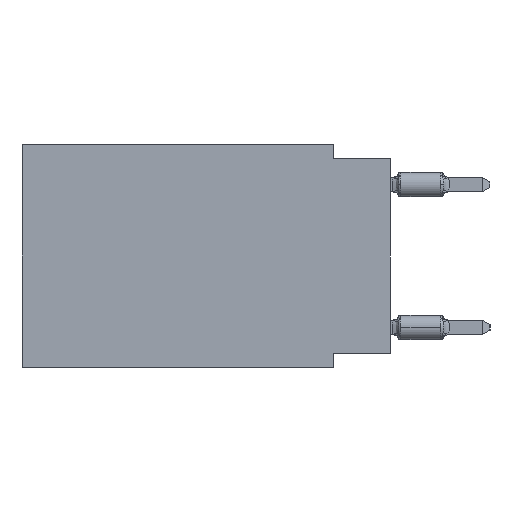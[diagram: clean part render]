
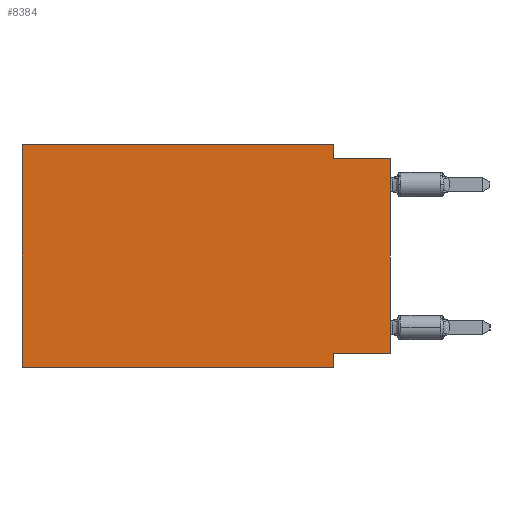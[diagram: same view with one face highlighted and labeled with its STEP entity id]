
A CAD part, left-side view. The second image highlights one B-rep face of the part: STEP entity #8384.
In plain terms, the highlighted planar face has unit normal (-1, 0, 0).
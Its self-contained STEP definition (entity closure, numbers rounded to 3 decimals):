
#720 = CARTESIAN_POINT ( 'NONE',  ( 0., 16.383, 0. ) ) ;
#1189 = VERTEX_POINT ( 'NONE', #13962 ) ;
#1485 = ORIENTED_EDGE ( 'NONE', *, *, #22149, .F. ) ;
#1695 = CARTESIAN_POINT ( 'NONE',  ( 0., 0., -0.635 ) ) ;
#2063 = ORIENTED_EDGE ( 'NONE', *, *, #5189, .F. ) ;
#2465 = CARTESIAN_POINT ( 'NONE',  ( 0., 2.54, 0. ) ) ;
#2857 = CARTESIAN_POINT ( 'NONE',  ( 0., 2.54, -9.906 ) ) ;
#2932 = VECTOR ( 'NONE', #26366, 1000. ) ;
#3085 = DIRECTION ( 'NONE',  ( 0., -1., 0. ) ) ;
#3864 = VECTOR ( 'NONE', #19333, 1000. ) ;
#5189 = EDGE_CURVE ( 'NONE', #25644, #33259, #33594, .T. ) ;
#5801 = AXIS2_PLACEMENT_3D ( 'NONE', #8804, #19275, #29767 ) ;
#5880 = ORIENTED_EDGE ( 'NONE', *, *, #22440, .T. ) ;
#6554 = LINE ( 'NONE', #14617, #33543 ) ;
#7058 = VERTEX_POINT ( 'NONE', #9525 ) ;
#7305 = EDGE_CURVE ( 'NONE', #1189, #25644, #24247, .T. ) ;
#8384 = ADVANCED_FACE ( 'NONE', ( #22182 ), #22357, .F. ) ;
#8414 = CARTESIAN_POINT ( 'NONE',  ( 0., 2.54, -9.271 ) ) ;
#8804 = CARTESIAN_POINT ( 'NONE',  ( 0., 16.383, 0. ) ) ;
#9525 = CARTESIAN_POINT ( 'NONE',  ( 0., 0., -9.271 ) ) ;
#11203 = DIRECTION ( 'NONE',  ( 0., -1., 0. ) ) ;
#11595 = VECTOR ( 'NONE', #3085, 1000. ) ;
#11649 = VERTEX_POINT ( 'NONE', #1695 ) ;
#11725 = VERTEX_POINT ( 'NONE', #29010 ) ;
#13463 = CARTESIAN_POINT ( 'NONE',  ( 0., 2.54, -9.906 ) ) ;
#13962 = CARTESIAN_POINT ( 'NONE',  ( 0., 16.383, 0. ) ) ;
#14617 = CARTESIAN_POINT ( 'NONE',  ( 0., 0., -9.271 ) ) ;
#14642 = CARTESIAN_POINT ( 'NONE',  ( 0., 2.54, 0. ) ) ;
#15489 = EDGE_CURVE ( 'NONE', #11725, #25548, #24831, .T. ) ;
#15730 = CARTESIAN_POINT ( 'NONE',  ( 0., 0., 0. ) ) ;
#17675 = EDGE_CURVE ( 'NONE', #7058, #17996, #6554, .T. ) ;
#17979 = EDGE_CURVE ( 'NONE', #33259, #11649, #27295, .T. ) ;
#17996 = VERTEX_POINT ( 'NONE', #8414 ) ;
#18061 = VECTOR ( 'NONE', #11203, 1000. ) ;
#18834 = CARTESIAN_POINT ( 'NONE',  ( 0., 16.383, 0. ) ) ;
#19242 = ORIENTED_EDGE ( 'NONE', *, *, #7305, .F. ) ;
#19275 = DIRECTION ( 'NONE',  ( 1., 0., 0. ) ) ;
#19333 = DIRECTION ( 'NONE',  ( 0., -1., 0. ) ) ;
#19519 = DIRECTION ( 'NONE',  ( 0., 0., 1. ) ) ;
#19674 = CARTESIAN_POINT ( 'NONE',  ( 0., 16.383, -9.906 ) ) ;
#19918 = VECTOR ( 'NONE', #19519, 1000. ) ;
#20026 = ORIENTED_EDGE ( 'NONE', *, *, #15489, .T. ) ;
#20875 = LINE ( 'NONE', #15730, #2932 ) ;
#21185 = DIRECTION ( 'NONE',  ( 0., 0., -1. ) ) ;
#22149 = EDGE_CURVE ( 'NONE', #11725, #1189, #32239, .T. ) ;
#22182 = FACE_OUTER_BOUND ( 'NONE', #28837, .T. ) ;
#22342 = DIRECTION ( 'NONE',  ( 0., 1., 0. ) ) ;
#22357 = PLANE ( 'NONE',  #5801 ) ;
#22440 = EDGE_CURVE ( 'NONE', #7058, #11649, #20875, .T. ) ;
#22764 = ORIENTED_EDGE ( 'NONE', *, *, #17675, .F. ) ;
#23157 = VECTOR ( 'NONE', #21185, 1000. ) ;
#24247 = LINE ( 'NONE', #720, #18061 ) ;
#24440 = VECTOR ( 'NONE', #30991, 1000. ) ;
#24831 = LINE ( 'NONE', #19674, #3864 ) ;
#25077 = ORIENTED_EDGE ( 'NONE', *, *, #27577, .F. ) ;
#25548 = VERTEX_POINT ( 'NONE', #2857 ) ;
#25644 = VERTEX_POINT ( 'NONE', #14642 ) ;
#26366 = DIRECTION ( 'NONE',  ( 0., 0., 1. ) ) ;
#27295 = LINE ( 'NONE', #32120, #11595 ) ;
#27577 = EDGE_CURVE ( 'NONE', #17996, #25548, #31349, .T. ) ;
#28837 = EDGE_LOOP ( 'NONE', ( #5880, #30894, #2063, #19242, #1485, #20026, #25077, #22764 ) ) ;
#29010 = CARTESIAN_POINT ( 'NONE',  ( 0., 16.383, -9.906 ) ) ;
#29767 = DIRECTION ( 'NONE',  ( 0., 0., -1. ) ) ;
#30894 = ORIENTED_EDGE ( 'NONE', *, *, #17979, .F. ) ;
#30991 = DIRECTION ( 'NONE',  ( 0., 0., -1. ) ) ;
#31132 = CARTESIAN_POINT ( 'NONE',  ( 0., 2.54, -0.635 ) ) ;
#31349 = LINE ( 'NONE', #13463, #23157 ) ;
#32120 = CARTESIAN_POINT ( 'NONE',  ( 0., 0., -0.635 ) ) ;
#32239 = LINE ( 'NONE', #18834, #19918 ) ;
#33259 = VERTEX_POINT ( 'NONE', #31132 ) ;
#33543 = VECTOR ( 'NONE', #22342, 1000. ) ;
#33594 = LINE ( 'NONE', #2465, #24440 ) ;
